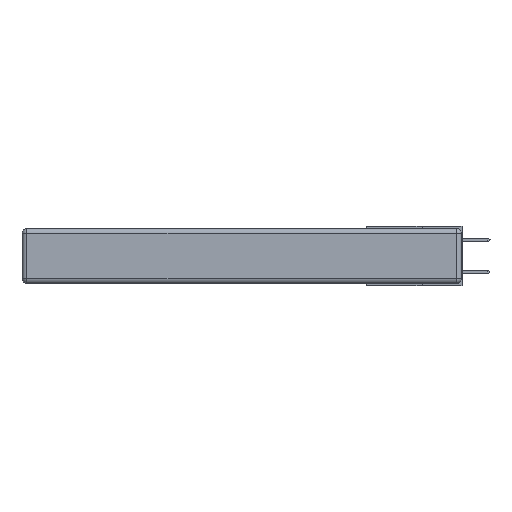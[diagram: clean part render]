
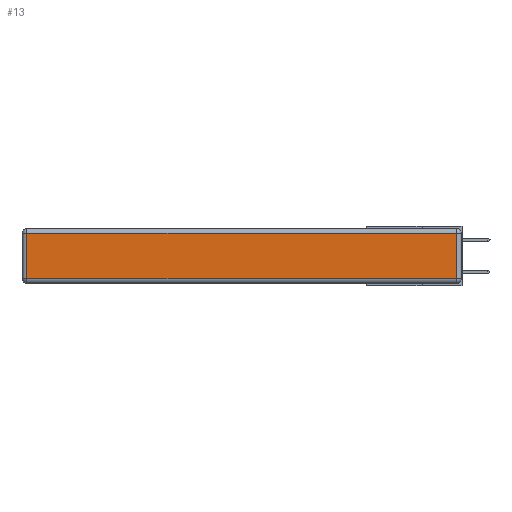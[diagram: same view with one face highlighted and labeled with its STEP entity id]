
A CAD part, left-side view. The second image highlights one B-rep face of the part: STEP entity #13.
In plain terms, the highlighted planar face has unit normal (-1, 0, 0).
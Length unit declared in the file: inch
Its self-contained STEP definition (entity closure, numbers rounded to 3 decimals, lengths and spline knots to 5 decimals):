
#13 = ADVANCED_FACE ( 'NONE', ( #4301 ), #2600, .T. ) ;
#423 = EDGE_CURVE ( 'NONE', #4318, #3833, #9150, .T. ) ;
#580 = CARTESIAN_POINT ( 'NONE',  ( 0., 0., -0.343 ) ) ;
#1076 = DIRECTION ( 'NONE',  ( 0., 1., 0. ) ) ;
#1753 = DIRECTION ( 'NONE',  ( -1., 0., 0. ) ) ;
#1915 = EDGE_CURVE ( 'NONE', #3833, #6481, #11397, .T. ) ;
#2261 = VECTOR ( 'NONE', #1076, 39.37008 ) ;
#2424 = ORIENTED_EDGE ( 'NONE', *, *, #1915, .T. ) ;
#2600 = PLANE ( 'NONE',  #4423 ) ;
#3254 = CARTESIAN_POINT ( 'NONE',  ( 0., 2.72, -0.313 ) ) ;
#3833 = VERTEX_POINT ( 'NONE', #10208 ) ;
#4301 = FACE_OUTER_BOUND ( 'NONE', #7817, .T. ) ;
#4318 = VERTEX_POINT ( 'NONE', #3254 ) ;
#4423 = AXIS2_PLACEMENT_3D ( 'NONE', #580, #1753, #10050 ) ;
#4623 = DIRECTION ( 'NONE',  ( 0., 0., 1. ) ) ;
#4638 = CARTESIAN_POINT ( 'NONE',  ( 0., 2.72, -0.343 ) ) ;
#4759 = LINE ( 'NONE', #4638, #7520 ) ;
#5200 = EDGE_CURVE ( 'NONE', #6481, #8119, #6989, .T. ) ;
#5698 = CARTESIAN_POINT ( 'NONE',  ( 0., 0.03, -0.343 ) ) ;
#6481 = VERTEX_POINT ( 'NONE', #7831 ) ;
#6989 = LINE ( 'NONE', #7290, #2261 ) ;
#7290 = CARTESIAN_POINT ( 'NONE',  ( 0., 2.75, -0.03 ) ) ;
#7520 = VECTOR ( 'NONE', #12847, 39.37008 ) ;
#7817 = EDGE_LOOP ( 'NONE', ( #10466, #2424, #9790, #11626 ) ) ;
#7831 = CARTESIAN_POINT ( 'NONE',  ( 0., 0.03, -0.03 ) ) ;
#7990 = CARTESIAN_POINT ( 'NONE',  ( 0., 2.72, -0.03 ) ) ;
#8119 = VERTEX_POINT ( 'NONE', #7990 ) ;
#8651 = VECTOR ( 'NONE', #4623, 39.37008 ) ;
#9150 = LINE ( 'NONE', #10536, #13380 ) ;
#9790 = ORIENTED_EDGE ( 'NONE', *, *, #5200, .T. ) ;
#10050 = DIRECTION ( 'NONE',  ( 0., 0., 1. ) ) ;
#10208 = CARTESIAN_POINT ( 'NONE',  ( 0., 0.03, -0.313 ) ) ;
#10466 = ORIENTED_EDGE ( 'NONE', *, *, #423, .T. ) ;
#10536 = CARTESIAN_POINT ( 'NONE',  ( 0., 0., -0.313 ) ) ;
#10578 = DIRECTION ( 'NONE',  ( 0., -1., 0. ) ) ;
#10759 = EDGE_CURVE ( 'NONE', #8119, #4318, #4759, .T. ) ;
#11397 = LINE ( 'NONE', #5698, #8651 ) ;
#11626 = ORIENTED_EDGE ( 'NONE', *, *, #10759, .T. ) ;
#12847 = DIRECTION ( 'NONE',  ( 0., 0., -1. ) ) ;
#13380 = VECTOR ( 'NONE', #10578, 39.37008 ) ;
